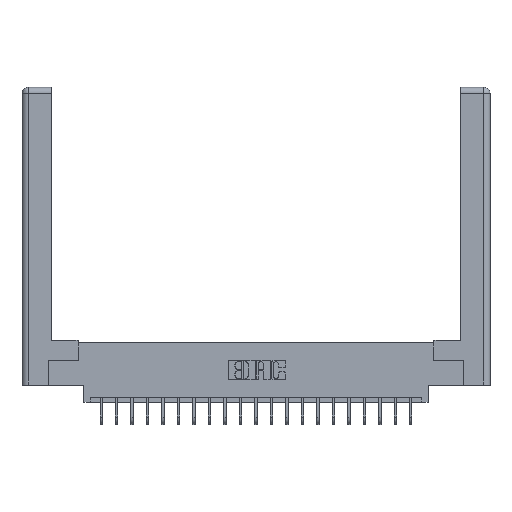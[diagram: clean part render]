
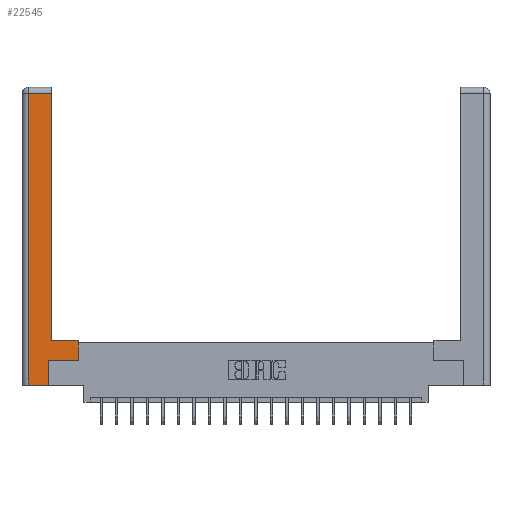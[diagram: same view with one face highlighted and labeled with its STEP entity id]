
A CAD part, top view. The second image highlights one B-rep face of the part: STEP entity #22545.
In plain terms, the highlighted planar face has unit normal (0, 0, 1).
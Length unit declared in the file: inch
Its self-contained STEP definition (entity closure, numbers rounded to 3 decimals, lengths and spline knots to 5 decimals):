
#102 = VERTEX_POINT ( 'NONE', #3297 ) ;
#161 = CARTESIAN_POINT ( 'NONE',  ( 0.0615, 2.94, 0. ) ) ;
#409 = EDGE_CURVE ( 'NONE', #102, #15671, #2057, .T. ) ;
#633 = ORIENTED_EDGE ( 'NONE', *, *, #9474, .T. ) ;
#714 = ORIENTED_EDGE ( 'NONE', *, *, #18338, .T. ) ;
#955 = VECTOR ( 'NONE', #12718, 39.37008 ) ;
#1329 = CARTESIAN_POINT ( 'NONE',  ( 0.295, 0.45, 0. ) ) ;
#1864 = VECTOR ( 'NONE', #9075, 39.37008 ) ;
#2050 = LINE ( 'NONE', #9812, #20826 ) ;
#2057 = LINE ( 'NONE', #6035, #17141 ) ;
#2203 = VERTEX_POINT ( 'NONE', #23451 ) ;
#2563 = ORIENTED_EDGE ( 'NONE', *, *, #409, .T. ) ;
#3197 = CARTESIAN_POINT ( 'NONE',  ( 0.565, 0.245, 0. ) ) ;
#3297 = CARTESIAN_POINT ( 'NONE',  ( 0.265, 0.245, 0. ) ) ;
#5596 = EDGE_CURVE ( 'NONE', #16134, #102, #11161, .T. ) ;
#5692 = DIRECTION ( 'NONE',  ( 0., 1., 0. ) ) ;
#6035 = CARTESIAN_POINT ( 'NONE',  ( 0.565, 0.245, 0. ) ) ;
#6205 = LINE ( 'NONE', #161, #18176 ) ;
#6575 = CARTESIAN_POINT ( 'NONE',  ( 0.295, 2.94, 0. ) ) ;
#6783 = AXIS2_PLACEMENT_3D ( 'NONE', #23515, #16449, #16529 ) ;
#7562 = CARTESIAN_POINT ( 'NONE',  ( 0.295, 0.45, 0. ) ) ;
#7571 = EDGE_LOOP ( 'NONE', ( #11079, #633, #14978, #14240, #20407, #2563, #714, #17535 ) ) ;
#8185 = EDGE_CURVE ( 'NONE', #11881, #10501, #17275, .T. ) ;
#8279 = CARTESIAN_POINT ( 'NONE',  ( 0.265, 0.245, 0. ) ) ;
#8640 = VERTEX_POINT ( 'NONE', #1329 ) ;
#8651 = DIRECTION ( 'NONE',  ( 0., -1., 0. ) ) ;
#9075 = DIRECTION ( 'NONE',  ( 1., 0., 0. ) ) ;
#9109 = VECTOR ( 'NONE', #5692, 39.37008 ) ;
#9474 = EDGE_CURVE ( 'NONE', #21296, #11881, #6205, .T. ) ;
#9698 = CARTESIAN_POINT ( 'NONE',  ( 0.0615, 2.94, 0. ) ) ;
#9812 = CARTESIAN_POINT ( 'NONE',  ( 0.565, 0.45, 0. ) ) ;
#10501 = VERTEX_POINT ( 'NONE', #11665 ) ;
#10926 = PLANE ( 'NONE',  #6783 ) ;
#11079 = ORIENTED_EDGE ( 'NONE', *, *, #21566, .T. ) ;
#11161 = LINE ( 'NONE', #8279, #14868 ) ;
#11540 = VECTOR ( 'NONE', #8651, 39.37008 ) ;
#11567 = DIRECTION ( 'NONE',  ( 0., 1., 0. ) ) ;
#11665 = CARTESIAN_POINT ( 'NONE',  ( 0.0615, 0., 0. ) ) ;
#11881 = VERTEX_POINT ( 'NONE', #9698 ) ;
#11903 = DIRECTION ( 'NONE',  ( 0., 1., 0. ) ) ;
#12718 = DIRECTION ( 'NONE',  ( -1., 0., 0. ) ) ;
#13685 = EDGE_CURVE ( 'NONE', #2203, #8640, #18060, .T. ) ;
#14240 = ORIENTED_EDGE ( 'NONE', *, *, #15126, .T. ) ;
#14868 = VECTOR ( 'NONE', #11903, 39.37008 ) ;
#14942 = DIRECTION ( 'NONE',  ( 1., 0., 0. ) ) ;
#14978 = ORIENTED_EDGE ( 'NONE', *, *, #8185, .T. ) ;
#15126 = EDGE_CURVE ( 'NONE', #10501, #16134, #15237, .T. ) ;
#15237 = LINE ( 'NONE', #19998, #1864 ) ;
#15671 = VERTEX_POINT ( 'NONE', #3197 ) ;
#16134 = VERTEX_POINT ( 'NONE', #17454 ) ;
#16449 = DIRECTION ( 'NONE',  ( 0., 0., -1. ) ) ;
#16529 = DIRECTION ( 'NONE',  ( -1., 0., 0. ) ) ;
#17141 = VECTOR ( 'NONE', #14942, 39.37008 ) ;
#17275 = LINE ( 'NONE', #19728, #11540 ) ;
#17454 = CARTESIAN_POINT ( 'NONE',  ( 0.265, 0., 0. ) ) ;
#17535 = ORIENTED_EDGE ( 'NONE', *, *, #13685, .T. ) ;
#18060 = LINE ( 'NONE', #7562, #955 ) ;
#18176 = VECTOR ( 'NONE', #22012, 39.37008 ) ;
#18338 = EDGE_CURVE ( 'NONE', #15671, #2203, #2050, .T. ) ;
#19728 = CARTESIAN_POINT ( 'NONE',  ( 0.0615, 0., 0. ) ) ;
#19925 = FACE_OUTER_BOUND ( 'NONE', #7571, .T. ) ;
#19998 = CARTESIAN_POINT ( 'NONE',  ( 0.265, 0., 0. ) ) ;
#20166 = CARTESIAN_POINT ( 'NONE',  ( 0.295, 3., 0. ) ) ;
#20407 = ORIENTED_EDGE ( 'NONE', *, *, #5596, .T. ) ;
#20826 = VECTOR ( 'NONE', #11567, 39.37008 ) ;
#21296 = VERTEX_POINT ( 'NONE', #6575 ) ;
#21566 = EDGE_CURVE ( 'NONE', #8640, #21296, #22465, .T. ) ;
#22012 = DIRECTION ( 'NONE',  ( -1., 0., 0. ) ) ;
#22465 = LINE ( 'NONE', #20166, #9109 ) ;
#22545 = ADVANCED_FACE ( 'NONE', ( #19925 ), #10926, .F. ) ;
#23451 = CARTESIAN_POINT ( 'NONE',  ( 0.565, 0.45, 0. ) ) ;
#23515 = CARTESIAN_POINT ( 'NONE',  ( 0., 0., 0. ) ) ;
